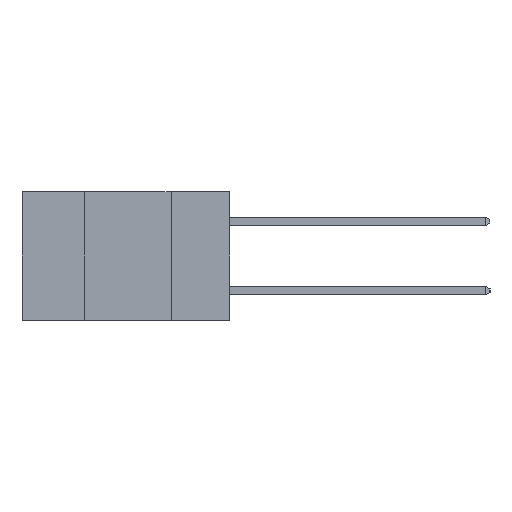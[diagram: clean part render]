
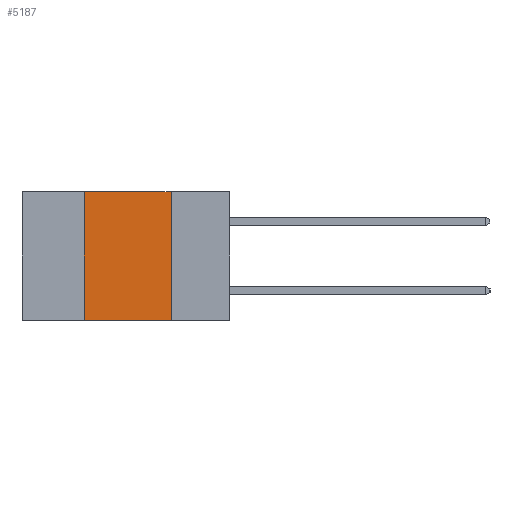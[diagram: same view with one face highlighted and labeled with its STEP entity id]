
A CAD part, left-side view. The second image highlights one B-rep face of the part: STEP entity #5187.
In plain terms, the highlighted planar face has unit normal (-1, 0, 0).
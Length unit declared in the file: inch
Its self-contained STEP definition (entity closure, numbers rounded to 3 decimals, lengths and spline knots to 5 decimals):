
#437 = CARTESIAN_POINT ( 'NONE',  ( 0., 0.6, -0.37 ) ) ;
#481 = CARTESIAN_POINT ( 'NONE',  ( 0., 0.17, 0. ) ) ;
#525 = ORIENTED_EDGE ( 'NONE', *, *, #12249, .F. ) ;
#688 = DIRECTION ( 'NONE',  ( 0., 0., 1. ) ) ;
#955 = ORIENTED_EDGE ( 'NONE', *, *, #1478, .T. ) ;
#1459 = CARTESIAN_POINT ( 'NONE',  ( 0., 0.6, 0. ) ) ;
#1478 = EDGE_CURVE ( 'NONE', #12481, #7542, #9982, .T. ) ;
#1549 = EDGE_CURVE ( 'NONE', #4094, #7542, #9024, .T. ) ;
#2071 = ORIENTED_EDGE ( 'NONE', *, *, #12661, .F. ) ;
#2473 = DIRECTION ( 'NONE',  ( 0., 0., -1. ) ) ;
#2725 = AXIS2_PLACEMENT_3D ( 'NONE', #1459, #8456, #2473 ) ;
#3128 = CARTESIAN_POINT ( 'NONE',  ( 0., 0.6, 0. ) ) ;
#3856 = VECTOR ( 'NONE', #7124, 39.37008 ) ;
#4094 = VERTEX_POINT ( 'NONE', #481 ) ;
#4494 = DIRECTION ( 'NONE',  ( 0., -1., 0. ) ) ;
#5177 = VERTEX_POINT ( 'NONE', #9433 ) ;
#5187 = ADVANCED_FACE ( 'NONE', ( #8449 ), #6457, .F. ) ;
#5485 = VECTOR ( 'NONE', #688, 39.37008 ) ;
#6367 = VECTOR ( 'NONE', #6574, 39.37008 ) ;
#6457 = PLANE ( 'NONE',  #2725 ) ;
#6574 = DIRECTION ( 'NONE',  ( 0., 0., -1. ) ) ;
#7124 = DIRECTION ( 'NONE',  ( 0., -1., 0. ) ) ;
#7305 = VECTOR ( 'NONE', #4494, 39.37008 ) ;
#7412 = CARTESIAN_POINT ( 'NONE',  ( 0., 0.42, -0.37 ) ) ;
#7542 = VERTEX_POINT ( 'NONE', #12403 ) ;
#7683 = CARTESIAN_POINT ( 'NONE',  ( 0., 0.42, -0.37 ) ) ;
#7962 = ORIENTED_EDGE ( 'NONE', *, *, #1549, .F. ) ;
#8449 = FACE_OUTER_BOUND ( 'NONE', #10413, .T. ) ;
#8456 = DIRECTION ( 'NONE',  ( 1., 0., 0. ) ) ;
#9024 = LINE ( 'NONE', #10520, #6367 ) ;
#9433 = CARTESIAN_POINT ( 'NONE',  ( 0., 0.42, 0. ) ) ;
#9982 = LINE ( 'NONE', #437, #7305 ) ;
#10413 = EDGE_LOOP ( 'NONE', ( #7962, #525, #2071, #955 ) ) ;
#10520 = CARTESIAN_POINT ( 'NONE',  ( 0., 0.17, -0.37 ) ) ;
#10812 = LINE ( 'NONE', #7683, #5485 ) ;
#11491 = LINE ( 'NONE', #3128, #3856 ) ;
#12249 = EDGE_CURVE ( 'NONE', #5177, #4094, #11491, .T. ) ;
#12403 = CARTESIAN_POINT ( 'NONE',  ( 0., 0.17, -0.37 ) ) ;
#12481 = VERTEX_POINT ( 'NONE', #7412 ) ;
#12661 = EDGE_CURVE ( 'NONE', #12481, #5177, #10812, .T. ) ;
